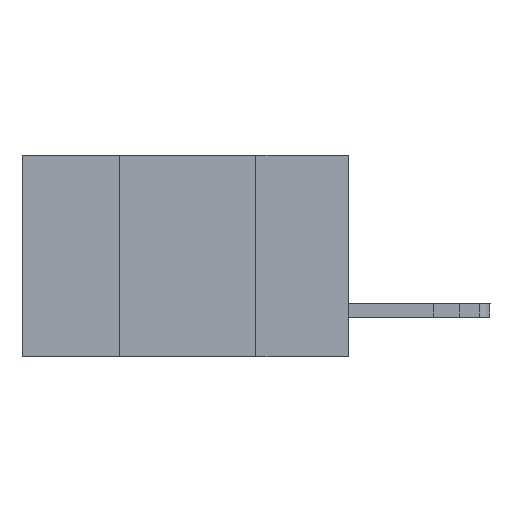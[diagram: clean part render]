
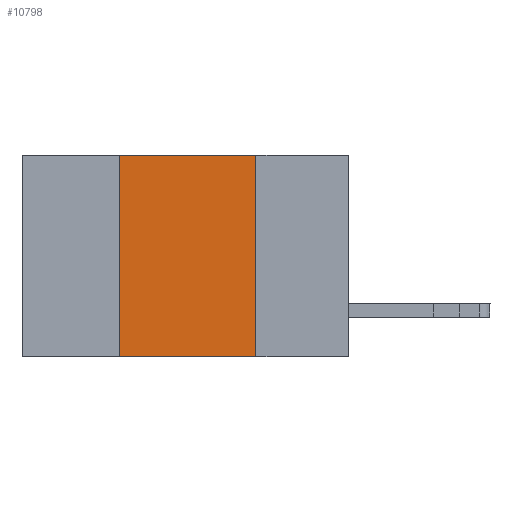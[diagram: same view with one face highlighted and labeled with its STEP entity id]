
A CAD part, left-side view. The second image highlights one B-rep face of the part: STEP entity #10798.
In plain terms, the highlighted planar face has unit normal (-1, 0, 0).
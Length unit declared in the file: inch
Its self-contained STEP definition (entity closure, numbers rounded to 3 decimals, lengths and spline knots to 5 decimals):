
#734 = VECTOR ( 'NONE', #6054, 39.37008 ) ;
#773 = DIRECTION ( 'NONE',  ( 1., 0., 0. ) ) ;
#795 = CARTESIAN_POINT ( 'NONE',  ( 0., 0.6, 0. ) ) ;
#1970 = ORIENTED_EDGE ( 'NONE', *, *, #8839, .F. ) ;
#2286 = CARTESIAN_POINT ( 'NONE',  ( 0., 0.17, -0.37 ) ) ;
#2644 = FACE_OUTER_BOUND ( 'NONE', #7016, .T. ) ;
#3205 = VERTEX_POINT ( 'NONE', #11079 ) ;
#3285 = DIRECTION ( 'NONE',  ( 0., -1., 0. ) ) ;
#3299 = LINE ( 'NONE', #795, #11395 ) ;
#3616 = ORIENTED_EDGE ( 'NONE', *, *, #4450, .F. ) ;
#4007 = VECTOR ( 'NONE', #3285, 39.37008 ) ;
#4163 = ORIENTED_EDGE ( 'NONE', *, *, #10350, .T. ) ;
#4450 = EDGE_CURVE ( 'NONE', #12011, #12289, #5811, .T. ) ;
#4998 = VECTOR ( 'NONE', #7353, 39.37008 ) ;
#5556 = CARTESIAN_POINT ( 'NONE',  ( 0., 0.42, 0. ) ) ;
#5769 = EDGE_CURVE ( 'NONE', #12289, #3205, #3299, .T. ) ;
#5811 = LINE ( 'NONE', #13695, #4998 ) ;
#6054 = DIRECTION ( 'NONE',  ( 0., 0., -1. ) ) ;
#7016 = EDGE_LOOP ( 'NONE', ( #1970, #10109, #3616, #4163 ) ) ;
#7353 = DIRECTION ( 'NONE',  ( 0., 0., 1. ) ) ;
#8163 = DIRECTION ( 'NONE',  ( 0., 0., -1. ) ) ;
#8498 = CARTESIAN_POINT ( 'NONE',  ( 0., 0.6, -0.37 ) ) ;
#8839 = EDGE_CURVE ( 'NONE', #3205, #13090, #9987, .T. ) ;
#9219 = DIRECTION ( 'NONE',  ( 0., -1., 0. ) ) ;
#9261 = CARTESIAN_POINT ( 'NONE',  ( 0., 0.17, -0.37 ) ) ;
#9925 = AXIS2_PLACEMENT_3D ( 'NONE', #10155, #773, #8163 ) ;
#9987 = LINE ( 'NONE', #9261, #734 ) ;
#10071 = CARTESIAN_POINT ( 'NONE',  ( 0., 0.42, -0.37 ) ) ;
#10109 = ORIENTED_EDGE ( 'NONE', *, *, #5769, .F. ) ;
#10155 = CARTESIAN_POINT ( 'NONE',  ( 0., 0.6, 0. ) ) ;
#10350 = EDGE_CURVE ( 'NONE', #12011, #13090, #12431, .T. ) ;
#10798 = ADVANCED_FACE ( 'NONE', ( #2644 ), #12360, .F. ) ;
#11079 = CARTESIAN_POINT ( 'NONE',  ( 0., 0.17, 0. ) ) ;
#11395 = VECTOR ( 'NONE', #9219, 39.37008 ) ;
#12011 = VERTEX_POINT ( 'NONE', #10071 ) ;
#12289 = VERTEX_POINT ( 'NONE', #5556 ) ;
#12360 = PLANE ( 'NONE',  #9925 ) ;
#12431 = LINE ( 'NONE', #8498, #4007 ) ;
#13090 = VERTEX_POINT ( 'NONE', #2286 ) ;
#13695 = CARTESIAN_POINT ( 'NONE',  ( 0., 0.42, -0.37 ) ) ;
